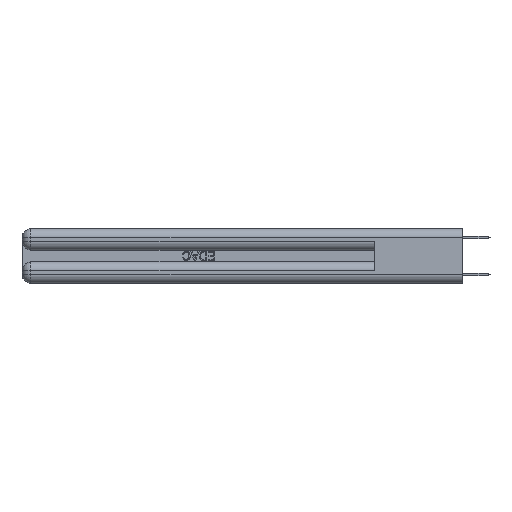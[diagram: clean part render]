
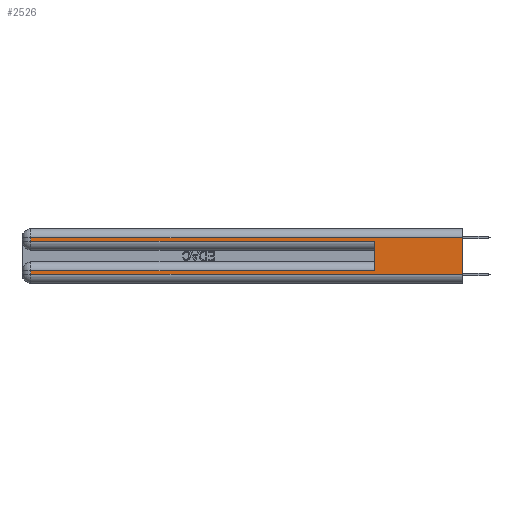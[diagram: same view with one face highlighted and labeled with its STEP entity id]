
A CAD part, left-side view. The second image highlights one B-rep face of the part: STEP entity #2526.
In plain terms, the highlighted planar face has unit normal (-1, 0, 0).
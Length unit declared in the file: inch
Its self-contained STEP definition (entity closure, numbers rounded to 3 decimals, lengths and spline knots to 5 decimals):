
#427 = LINE ( 'NONE', #16865, #27180 ) ;
#557 = VERTEX_POINT ( 'NONE', #3459 ) ;
#616 = EDGE_CURVE ( 'NONE', #13582, #3377, #29296, .T. ) ;
#926 = EDGE_CURVE ( 'NONE', #7903, #27262, #15119, .T. ) ;
#2202 = CARTESIAN_POINT ( 'NONE',  ( 0., 0., 0.31 ) ) ;
#2520 = ORIENTED_EDGE ( 'NONE', *, *, #28713, .F. ) ;
#2526 = ADVANCED_FACE ( 'NONE', ( #18881 ), #28040, .F. ) ;
#3377 = VERTEX_POINT ( 'NONE', #11352 ) ;
#3459 = CARTESIAN_POINT ( 'NONE',  ( 0., 0., 0.06 ) ) ;
#3601 = DIRECTION ( 'NONE',  ( 0., 0., 1. ) ) ;
#3812 = LINE ( 'NONE', #24179, #5220 ) ;
#3955 = CARTESIAN_POINT ( 'NONE',  ( 0., 2.94, 0.085 ) ) ;
#4375 = EDGE_CURVE ( 'NONE', #16615, #13582, #427, .T. ) ;
#4696 = CARTESIAN_POINT ( 'NONE',  ( 0., 2.94, 0.31 ) ) ;
#4920 = DIRECTION ( 'NONE',  ( 1., 0., 0. ) ) ;
#5136 = VECTOR ( 'NONE', #5393, 39.37008 ) ;
#5220 = VECTOR ( 'NONE', #19901, 39.37008 ) ;
#5282 = DIRECTION ( 'NONE',  ( 0., -1., 0. ) ) ;
#5393 = DIRECTION ( 'NONE',  ( 0., 0., -1. ) ) ;
#6894 = VERTEX_POINT ( 'NONE', #4696 ) ;
#7480 = ORIENTED_EDGE ( 'NONE', *, *, #21694, .F. ) ;
#7903 = VERTEX_POINT ( 'NONE', #27085 ) ;
#8897 = CARTESIAN_POINT ( 'NONE',  ( 0., 2.94, 0.37 ) ) ;
#10072 = EDGE_CURVE ( 'NONE', #21884, #6894, #25300, .T. ) ;
#11352 = CARTESIAN_POINT ( 'NONE',  ( 0., 2.94, 0.06 ) ) ;
#11874 = VECTOR ( 'NONE', #5282, 39.37008 ) ;
#12147 = EDGE_LOOP ( 'NONE', ( #7480, #23535, #16923, #16754, #2520, #19656, #14360, #18579 ) ) ;
#13582 = VERTEX_POINT ( 'NONE', #3955 ) ;
#14292 = VECTOR ( 'NONE', #26223, 39.37008 ) ;
#14360 = ORIENTED_EDGE ( 'NONE', *, *, #616, .T. ) ;
#15119 = LINE ( 'NONE', #21955, #14292 ) ;
#16615 = VERTEX_POINT ( 'NONE', #27829 ) ;
#16754 = ORIENTED_EDGE ( 'NONE', *, *, #926, .T. ) ;
#16865 = CARTESIAN_POINT ( 'NONE',  ( 0., 0., 0.085 ) ) ;
#16923 = ORIENTED_EDGE ( 'NONE', *, *, #23670, .T. ) ;
#17378 = VECTOR ( 'NONE', #27906, 39.37008 ) ;
#18134 = CARTESIAN_POINT ( 'NONE',  ( 0., 0., 0.31 ) ) ;
#18528 = EDGE_CURVE ( 'NONE', #3377, #557, #28558, .T. ) ;
#18579 = ORIENTED_EDGE ( 'NONE', *, *, #18528, .T. ) ;
#18881 = FACE_OUTER_BOUND ( 'NONE', #12147, .T. ) ;
#19125 = DIRECTION ( 'NONE',  ( 0., 1., 0. ) ) ;
#19656 = ORIENTED_EDGE ( 'NONE', *, *, #4375, .T. ) ;
#19901 = DIRECTION ( 'NONE',  ( 0., 0., -1. ) ) ;
#21694 = EDGE_CURVE ( 'NONE', #21884, #557, #28521, .T. ) ;
#21884 = VERTEX_POINT ( 'NONE', #18134 ) ;
#21898 = VECTOR ( 'NONE', #3601, 39.37008 ) ;
#21955 = CARTESIAN_POINT ( 'NONE',  ( 0., 0., 0.285 ) ) ;
#22738 = DIRECTION ( 'NONE',  ( 0., 0., -1. ) ) ;
#23166 = DIRECTION ( 'NONE',  ( 0., 0., -1. ) ) ;
#23535 = ORIENTED_EDGE ( 'NONE', *, *, #10072, .T. ) ;
#23633 = CARTESIAN_POINT ( 'NONE',  ( 0., 0., 0.37 ) ) ;
#23665 = CARTESIAN_POINT ( 'NONE',  ( 0., 0., 0.06 ) ) ;
#23670 = EDGE_CURVE ( 'NONE', #6894, #7903, #3812, .T. ) ;
#24179 = CARTESIAN_POINT ( 'NONE',  ( 0., 2.94, 0.37 ) ) ;
#24885 = AXIS2_PLACEMENT_3D ( 'NONE', #25882, #4920, #23166 ) ;
#25300 = LINE ( 'NONE', #2202, #17378 ) ;
#25882 = CARTESIAN_POINT ( 'NONE',  ( 0., 0., 0.37 ) ) ;
#26223 = DIRECTION ( 'NONE',  ( 0., -1., 0. ) ) ;
#27085 = CARTESIAN_POINT ( 'NONE',  ( 0., 2.94, 0.285 ) ) ;
#27164 = LINE ( 'NONE', #28999, #21898 ) ;
#27180 = VECTOR ( 'NONE', #19125, 39.37008 ) ;
#27262 = VERTEX_POINT ( 'NONE', #28236 ) ;
#27829 = CARTESIAN_POINT ( 'NONE',  ( 0., 0.6, 0.085 ) ) ;
#27906 = DIRECTION ( 'NONE',  ( 0., 1., 0. ) ) ;
#28040 = PLANE ( 'NONE',  #24885 ) ;
#28236 = CARTESIAN_POINT ( 'NONE',  ( 0., 0.6, 0.285 ) ) ;
#28521 = LINE ( 'NONE', #23633, #5136 ) ;
#28558 = LINE ( 'NONE', #23665, #11874 ) ;
#28713 = EDGE_CURVE ( 'NONE', #16615, #27262, #27164, .T. ) ;
#28829 = VECTOR ( 'NONE', #22738, 39.37008 ) ;
#28999 = CARTESIAN_POINT ( 'NONE',  ( 0., 0.6, 0.145 ) ) ;
#29296 = LINE ( 'NONE', #8897, #28829 ) ;
